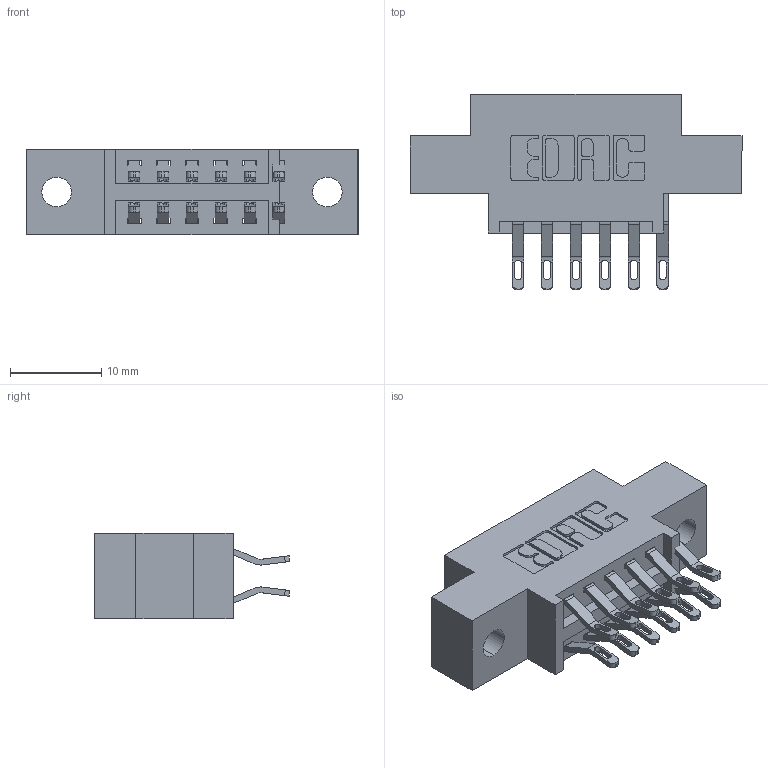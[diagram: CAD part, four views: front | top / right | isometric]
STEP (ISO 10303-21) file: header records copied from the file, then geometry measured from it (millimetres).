
FILE_DESCRIPTION (( 'STEP AP203' ), '1' );
FILE_NAME ('346-012-555-802.STEP', '2022-05-17T20:23:04', ( '' ), ( '' ), 'SwSTEP 2.0', 'SolidWorks 2020', '' );
FILE_SCHEMA (( 'CONFIG_CONTROL_DESIGN' ));
Length unit declared in the file: inch
Products named in the file (3): 345-292-001_555 Tail; 346-012-555-802; 346 Part_0.170 Offset - 0.128 Dia
Assembly tree (13 placements, depth 2):
  346-012-555-802
    346 Part_0.170 Offset - 0.128 Dia
    345-292-001_555 Tail  x12
Bounding box: 36.45 x 21.46 x 9.4 mm (x, y, z)
Volume: 3128.4 mm3; surface area: 3856.8 mm2
Topology: 13 solids, 13 shells, 810 faces, 2495 edges, 1662 vertices
Faces by surface type: plane 466, cylinder 344
Entity records: 8769 total; most frequent: CARTESIAN_POINT 1524, ORIENTED_EDGE 1426, DIRECTION 1365, EDGE_CURVE 713, LINE 541, VECTOR 541, VERTEX_POINT 474, AXIS2_PLACEMENT_3D 412
